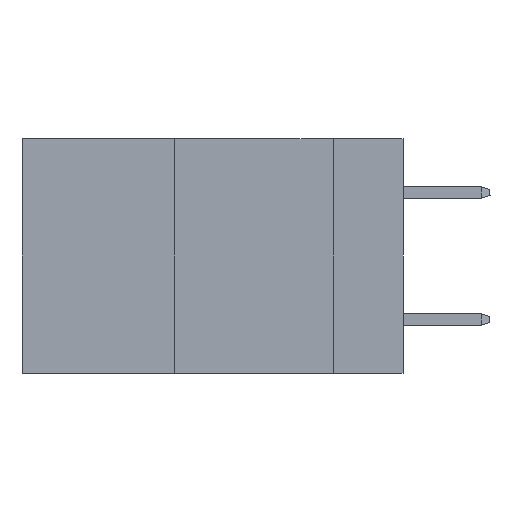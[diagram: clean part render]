
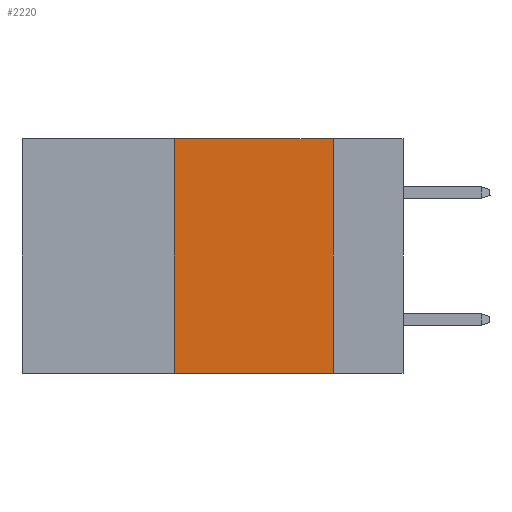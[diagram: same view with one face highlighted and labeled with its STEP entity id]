
A CAD part, left-side view. The second image highlights one B-rep face of the part: STEP entity #2220.
In plain terms, the highlighted planar face has unit normal (-1, 0, 0).
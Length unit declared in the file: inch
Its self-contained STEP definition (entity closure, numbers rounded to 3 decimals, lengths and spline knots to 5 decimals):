
#434 = ORIENTED_EDGE ( 'NONE', *, *, #7916, .F. ) ;
#609 = LINE ( 'NONE', #10777, #20897 ) ;
#2121 = AXIS2_PLACEMENT_3D ( 'NONE', #3788, #7761, #10400 ) ;
#2220 = ADVANCED_FACE ( 'NONE', ( #37877 ), #20524, .F. ) ;
#2572 = VERTEX_POINT ( 'NONE', #14311 ) ;
#3788 = CARTESIAN_POINT ( 'NONE',  ( 0., 0.6, 0. ) ) ;
#5562 = LINE ( 'NONE', #33601, #40974 ) ;
#6618 = DIRECTION ( 'NONE',  ( 0., -1., 0. ) ) ;
#6742 = VECTOR ( 'NONE', #6618, 39.37008 ) ;
#7761 = DIRECTION ( 'NONE',  ( 1., 0., 0. ) ) ;
#7916 = EDGE_CURVE ( 'NONE', #39042, #2572, #11483, .T. ) ;
#9632 = EDGE_CURVE ( 'NONE', #11986, #39042, #609, .T. ) ;
#10400 = DIRECTION ( 'NONE',  ( 0., 0., -1. ) ) ;
#10777 = CARTESIAN_POINT ( 'NONE',  ( 0., 0.6, 0. ) ) ;
#11065 = CARTESIAN_POINT ( 'NONE',  ( 0., 0.36, -0.37 ) ) ;
#11483 = LINE ( 'NONE', #24872, #23704 ) ;
#11986 = VERTEX_POINT ( 'NONE', #17952 ) ;
#12929 = EDGE_LOOP ( 'NONE', ( #434, #25891, #35552, #24609 ) ) ;
#13657 = CARTESIAN_POINT ( 'NONE',  ( 0., 0.6, -0.37 ) ) ;
#14311 = CARTESIAN_POINT ( 'NONE',  ( 0., 0.11, -0.37 ) ) ;
#17906 = EDGE_CURVE ( 'NONE', #29282, #11986, #5562, .T. ) ;
#17952 = CARTESIAN_POINT ( 'NONE',  ( 0., 0.36, 0. ) ) ;
#20524 = PLANE ( 'NONE',  #2121 ) ;
#20897 = VECTOR ( 'NONE', #38241, 39.37008 ) ;
#23704 = VECTOR ( 'NONE', #29017, 39.37008 ) ;
#24609 = ORIENTED_EDGE ( 'NONE', *, *, #36063, .T. ) ;
#24872 = CARTESIAN_POINT ( 'NONE',  ( 0., 0.11, 0. ) ) ;
#25891 = ORIENTED_EDGE ( 'NONE', *, *, #9632, .F. ) ;
#28175 = CARTESIAN_POINT ( 'NONE',  ( 0., 0.11, 0. ) ) ;
#29017 = DIRECTION ( 'NONE',  ( 0., 0., -1. ) ) ;
#29282 = VERTEX_POINT ( 'NONE', #11065 ) ;
#33601 = CARTESIAN_POINT ( 'NONE',  ( 0., 0.36, 0. ) ) ;
#35552 = ORIENTED_EDGE ( 'NONE', *, *, #17906, .F. ) ;
#36063 = EDGE_CURVE ( 'NONE', #29282, #2572, #37154, .T. ) ;
#37154 = LINE ( 'NONE', #13657, #6742 ) ;
#37877 = FACE_OUTER_BOUND ( 'NONE', #12929, .T. ) ;
#38241 = DIRECTION ( 'NONE',  ( 0., -1., 0. ) ) ;
#39042 = VERTEX_POINT ( 'NONE', #28175 ) ;
#40974 = VECTOR ( 'NONE', #42510, 39.37008 ) ;
#42510 = DIRECTION ( 'NONE',  ( 0., 0., 1. ) ) ;
